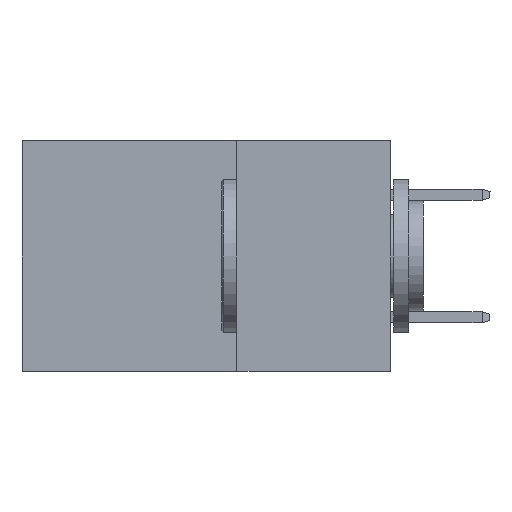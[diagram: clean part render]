
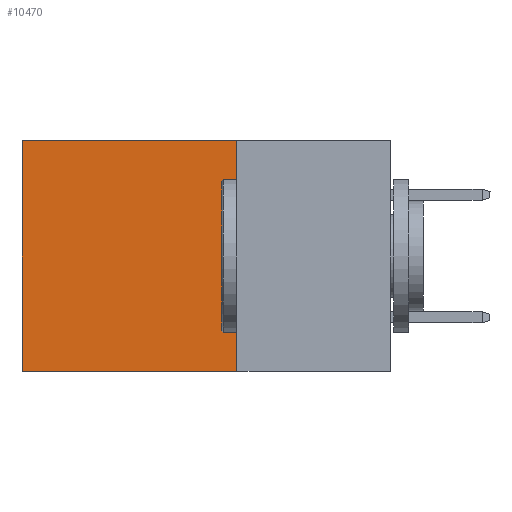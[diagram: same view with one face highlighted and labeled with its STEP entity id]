
A CAD part, left-side view. The second image highlights one B-rep face of the part: STEP entity #10470.
In plain terms, the highlighted planar face has unit normal (-1, 0, 0).
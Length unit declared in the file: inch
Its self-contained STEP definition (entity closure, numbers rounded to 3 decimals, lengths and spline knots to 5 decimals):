
#121 = ORIENTED_EDGE ( 'NONE', *, *, #10748, .F. ) ;
#530 = VECTOR ( 'NONE', #12022, 39.37008 ) ;
#882 = ORIENTED_EDGE ( 'NONE', *, *, #13632, .T. ) ;
#1015 = LINE ( 'NONE', #4129, #12850 ) ;
#1180 = PLANE ( 'NONE',  #3531 ) ;
#1260 = DIRECTION ( 'NONE',  ( 1., 0., 0. ) ) ;
#1401 = DIRECTION ( 'NONE',  ( 0., 0., -1. ) ) ;
#1908 = DIRECTION ( 'NONE',  ( 0., 0., -1. ) ) ;
#2290 = VERTEX_POINT ( 'NONE', #9941 ) ;
#3531 = AXIS2_PLACEMENT_3D ( 'NONE', #5763, #1260, #1401 ) ;
#3775 = ORIENTED_EDGE ( 'NONE', *, *, #12122, .T. ) ;
#3845 = VERTEX_POINT ( 'NONE', #4888 ) ;
#4129 = CARTESIAN_POINT ( 'NONE',  ( 0.2875, 0.25, 0. ) ) ;
#4594 = EDGE_CURVE ( 'NONE', #3845, #2290, #8048, .T. ) ;
#4866 = VERTEX_POINT ( 'NONE', #7456 ) ;
#4888 = CARTESIAN_POINT ( 'NONE',  ( 0.2875, 0.25, -0.375 ) ) ;
#5376 = DIRECTION ( 'NONE',  ( 0., 1., 0. ) ) ;
#5763 = CARTESIAN_POINT ( 'NONE',  ( 0.2875, 0.25, -0.375 ) ) ;
#6812 = DIRECTION ( 'NONE',  ( 0., 1., 0. ) ) ;
#6998 = VECTOR ( 'NONE', #1908, 39.37008 ) ;
#7395 = VERTEX_POINT ( 'NONE', #12629 ) ;
#7456 = CARTESIAN_POINT ( 'NONE',  ( 0.2875, 0.25, 0. ) ) ;
#7570 = CARTESIAN_POINT ( 'NONE',  ( 0.2875, 0.25, -0.375 ) ) ;
#8048 = LINE ( 'NONE', #12503, #8888 ) ;
#8888 = VECTOR ( 'NONE', #6812, 39.37008 ) ;
#9941 = CARTESIAN_POINT ( 'NONE',  ( 0.2875, 0.6, -0.375 ) ) ;
#10470 = ADVANCED_FACE ( 'NONE', ( #11307 ), #1180, .F. ) ;
#10748 = EDGE_CURVE ( 'NONE', #4866, #3845, #12984, .T. ) ;
#11307 = FACE_OUTER_BOUND ( 'NONE', #12972, .T. ) ;
#11878 = CARTESIAN_POINT ( 'NONE',  ( 0.2875, 0.6, -0.375 ) ) ;
#12022 = DIRECTION ( 'NONE',  ( 0., 0., -1. ) ) ;
#12122 = EDGE_CURVE ( 'NONE', #4866, #7395, #1015, .T. ) ;
#12503 = CARTESIAN_POINT ( 'NONE',  ( 0.2875, 0.25, -0.375 ) ) ;
#12629 = CARTESIAN_POINT ( 'NONE',  ( 0.2875, 0.6, 0. ) ) ;
#12850 = VECTOR ( 'NONE', #5376, 39.37008 ) ;
#12972 = EDGE_LOOP ( 'NONE', ( #882, #13419, #121, #3775 ) ) ;
#12984 = LINE ( 'NONE', #7570, #530 ) ;
#12988 = LINE ( 'NONE', #11878, #6998 ) ;
#13419 = ORIENTED_EDGE ( 'NONE', *, *, #4594, .F. ) ;
#13632 = EDGE_CURVE ( 'NONE', #7395, #2290, #12988, .T. ) ;
